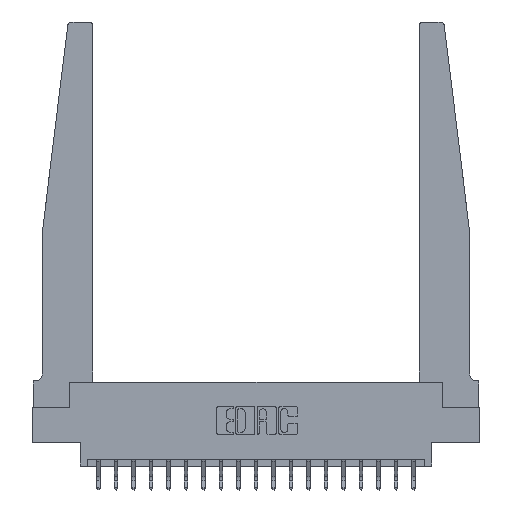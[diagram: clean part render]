
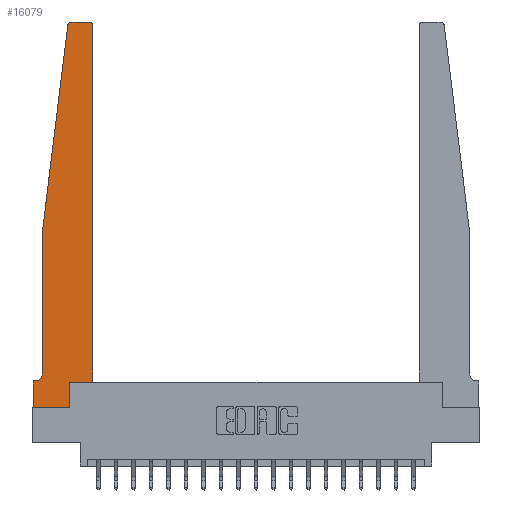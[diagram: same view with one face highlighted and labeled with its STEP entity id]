
A CAD part, top view. The second image highlights one B-rep face of the part: STEP entity #16079.
In plain terms, the highlighted planar face has unit normal (0, 0, 1).
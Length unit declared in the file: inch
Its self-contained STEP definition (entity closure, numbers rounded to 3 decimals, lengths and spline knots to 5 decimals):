
#51 = DIRECTION ( 'NONE',  ( 0., 0., 1. ) ) ;
#323 = VERTEX_POINT ( 'NONE', #16278 ) ;
#373 = CARTESIAN_POINT ( 'NONE',  ( 0.015, 0.1875, 0.37 ) ) ;
#1283 = DIRECTION ( 'NONE',  ( 1., 0., 0. ) ) ;
#1300 = CARTESIAN_POINT ( 'NONE',  ( 0.425, 0.18, 0.37 ) ) ;
#1454 = CIRCLE ( 'NONE', #8989, 0.03 ) ;
#1874 = ORIENTED_EDGE ( 'NONE', *, *, #9507, .T. ) ;
#1940 = LINE ( 'NONE', #7197, #2160 ) ;
#2062 = DIRECTION ( 'NONE',  ( 0., -1., 0. ) ) ;
#2160 = VECTOR ( 'NONE', #12111, 39.37008 ) ;
#2694 = DIRECTION ( 'NONE',  ( 1., 0., 0. ) ) ;
#2806 = ORIENTED_EDGE ( 'NONE', *, *, #17323, .T. ) ;
#2855 = VERTEX_POINT ( 'NONE', #19592 ) ;
#2858 = LINE ( 'NONE', #7587, #15596 ) ;
#3519 = VERTEX_POINT ( 'NONE', #19095 ) ;
#3650 = ORIENTED_EDGE ( 'NONE', *, *, #14130, .T. ) ;
#3895 = LINE ( 'NONE', #11901, #10871 ) ;
#4510 = CARTESIAN_POINT ( 'NONE',  ( 0.395, 2.72, 0.37 ) ) ;
#4593 = PLANE ( 'NONE',  #15401 ) ;
#5065 = CARTESIAN_POINT ( 'NONE',  ( 0.2605, 0.18, 0.37 ) ) ;
#5073 = VERTEX_POINT ( 'NONE', #16963 ) ;
#5094 = ORIENTED_EDGE ( 'NONE', *, *, #12721, .T. ) ;
#5113 = VERTEX_POINT ( 'NONE', #7181 ) ;
#5264 = DIRECTION ( 'NONE',  ( 1., 0., 0. ) ) ;
#5990 = DIRECTION ( 'NONE',  ( -1., 0., 0. ) ) ;
#6297 = LINE ( 'NONE', #19589, #11947 ) ;
#6327 = EDGE_CURVE ( 'NONE', #3519, #14732, #3895, .T. ) ;
#7137 = VECTOR ( 'NONE', #2694, 39.37008 ) ;
#7181 = CARTESIAN_POINT ( 'NONE',  ( 0.065, 0.2375, 0.37 ) ) ;
#7197 = CARTESIAN_POINT ( 'NONE',  ( 0.065, 1.25, 0.37 ) ) ;
#7543 = VERTEX_POINT ( 'NONE', #9309 ) ;
#7587 = CARTESIAN_POINT ( 'NONE',  ( 0.065, 0.1875, 0.37 ) ) ;
#7635 = LINE ( 'NONE', #1300, #8517 ) ;
#8074 = DIRECTION ( 'NONE',  ( 1., 0., 0. ) ) ;
#8454 = VERTEX_POINT ( 'NONE', #17507 ) ;
#8517 = VECTOR ( 'NONE', #14315, 39.37008 ) ;
#8763 = ORIENTED_EDGE ( 'NONE', *, *, #6327, .T. ) ;
#8989 = AXIS2_PLACEMENT_3D ( 'NONE', #4510, #19089, #1283 ) ;
#9309 = CARTESIAN_POINT ( 'NONE',  ( 0.27653, 2.75, 0.37 ) ) ;
#9418 = EDGE_CURVE ( 'NONE', #17878, #3519, #2858, .T. ) ;
#9507 = EDGE_CURVE ( 'NONE', #5113, #17878, #14553, .T. ) ;
#9602 = DIRECTION ( 'NONE',  ( 0., 0., 1. ) ) ;
#9710 = FACE_OUTER_BOUND ( 'NONE', #18043, .T. ) ;
#9809 = CARTESIAN_POINT ( 'NONE',  ( 0.015, 0.2375, 0.37 ) ) ;
#9815 = DIRECTION ( 'NONE',  ( 1., 0., 0. ) ) ;
#10334 = ORIENTED_EDGE ( 'NONE', *, *, #12886, .T. ) ;
#10481 = DIRECTION ( 'NONE',  ( 0., 1., 0. ) ) ;
#10748 = EDGE_CURVE ( 'NONE', #14732, #323, #18998, .T. ) ;
#10871 = VECTOR ( 'NONE', #2062, 39.37008 ) ;
#11481 = ORIENTED_EDGE ( 'NONE', *, *, #19610, .T. ) ;
#11670 = CARTESIAN_POINT ( 'NONE',  ( 0.425, 2.72, 0.37 ) ) ;
#11800 = CARTESIAN_POINT ( 'NONE',  ( 0.27653, 2.72, 0.37 ) ) ;
#11893 = LINE ( 'NONE', #18259, #15443 ) ;
#11898 = EDGE_CURVE ( 'NONE', #5073, #13220, #7635, .T. ) ;
#11901 = CARTESIAN_POINT ( 'NONE',  ( 0., 0., 0.37 ) ) ;
#11947 = VECTOR ( 'NONE', #17772, 39.37008 ) ;
#12007 = DIRECTION ( 'NONE',  ( -1., 0., 0. ) ) ;
#12011 = DIRECTION ( 'NONE',  ( -1., 0., 0. ) ) ;
#12111 = DIRECTION ( 'NONE',  ( 0., -1., 0. ) ) ;
#12721 = EDGE_CURVE ( 'NONE', #323, #13159, #15152, .T. ) ;
#12886 = EDGE_CURVE ( 'NONE', #7543, #2855, #15952, .T. ) ;
#12908 = VECTOR ( 'NONE', #10481, 39.37008 ) ;
#13159 = VERTEX_POINT ( 'NONE', #5065 ) ;
#13220 = VERTEX_POINT ( 'NONE', #11670 ) ;
#13343 = LINE ( 'NONE', #19831, #15141 ) ;
#13560 = CARTESIAN_POINT ( 'NONE',  ( 0.2605, 0.18, 0.37 ) ) ;
#13861 = CARTESIAN_POINT ( 'NONE',  ( 0., 0., 0.37 ) ) ;
#14130 = EDGE_CURVE ( 'NONE', #2855, #8454, #6297, .T. ) ;
#14185 = VERTEX_POINT ( 'NONE', #14475 ) ;
#14315 = DIRECTION ( 'NONE',  ( 0., 1., 0. ) ) ;
#14475 = CARTESIAN_POINT ( 'NONE',  ( 0.395, 2.75, 0.37 ) ) ;
#14553 = CIRCLE ( 'NONE', #19308, 0.05 ) ;
#14732 = VERTEX_POINT ( 'NONE', #13861 ) ;
#15141 = VECTOR ( 'NONE', #5264, 39.37008 ) ;
#15152 = LINE ( 'NONE', #13560, #12908 ) ;
#15401 = AXIS2_PLACEMENT_3D ( 'NONE', #17566, #9602, #9815 ) ;
#15443 = VECTOR ( 'NONE', #12007, 39.37008 ) ;
#15596 = VECTOR ( 'NONE', #5990, 39.37008 ) ;
#15952 = CIRCLE ( 'NONE', #16309, 0.03 ) ;
#16079 = ADVANCED_FACE ( 'NONE', ( #9710 ), #4593, .T. ) ;
#16278 = CARTESIAN_POINT ( 'NONE',  ( 0.2605, 0., 0.37 ) ) ;
#16309 = AXIS2_PLACEMENT_3D ( 'NONE', #11800, #51, #8074 ) ;
#16963 = CARTESIAN_POINT ( 'NONE',  ( 0.425, 0.18, 0.37 ) ) ;
#17235 = ORIENTED_EDGE ( 'NONE', *, *, #11898, .T. ) ;
#17323 = EDGE_CURVE ( 'NONE', #13220, #14185, #1454, .T. ) ;
#17507 = CARTESIAN_POINT ( 'NONE',  ( 0.065, 1.25, 0.37 ) ) ;
#17566 = CARTESIAN_POINT ( 'NONE',  ( 0., 0.1875, 0.37 ) ) ;
#17772 = DIRECTION ( 'NONE',  ( -0.122, -0.992, 0. ) ) ;
#17874 = DIRECTION ( 'NONE',  ( 0., 0., -1. ) ) ;
#17878 = VERTEX_POINT ( 'NONE', #373 ) ;
#18043 = EDGE_LOOP ( 'NONE', ( #11481, #10334, #3650, #18509, #1874, #19894, #8763, #21020, #5094, #19314, #17235, #2806 ) ) ;
#18259 = CARTESIAN_POINT ( 'NONE',  ( 0.25, 2.75, 0.37 ) ) ;
#18367 = EDGE_CURVE ( 'NONE', #8454, #5113, #1940, .T. ) ;
#18509 = ORIENTED_EDGE ( 'NONE', *, *, #18367, .T. ) ;
#18832 = EDGE_CURVE ( 'NONE', #13159, #5073, #13343, .T. ) ;
#18998 = LINE ( 'NONE', #20704, #7137 ) ;
#19089 = DIRECTION ( 'NONE',  ( 0., 0., 1. ) ) ;
#19095 = CARTESIAN_POINT ( 'NONE',  ( 0., 0.1875, 0.37 ) ) ;
#19308 = AXIS2_PLACEMENT_3D ( 'NONE', #9809, #17874, #12011 ) ;
#19314 = ORIENTED_EDGE ( 'NONE', *, *, #18832, .T. ) ;
#19589 = CARTESIAN_POINT ( 'NONE',  ( 0.065, 1.25, 0.37 ) ) ;
#19592 = CARTESIAN_POINT ( 'NONE',  ( 0.24675, 2.72367, 0.37 ) ) ;
#19610 = EDGE_CURVE ( 'NONE', #14185, #7543, #11893, .T. ) ;
#19831 = CARTESIAN_POINT ( 'NONE',  ( 0.425, 0.18, 0.37 ) ) ;
#19894 = ORIENTED_EDGE ( 'NONE', *, *, #9418, .T. ) ;
#20704 = CARTESIAN_POINT ( 'NONE',  ( 0., 0., 0.37 ) ) ;
#21020 = ORIENTED_EDGE ( 'NONE', *, *, #10748, .T. ) ;
